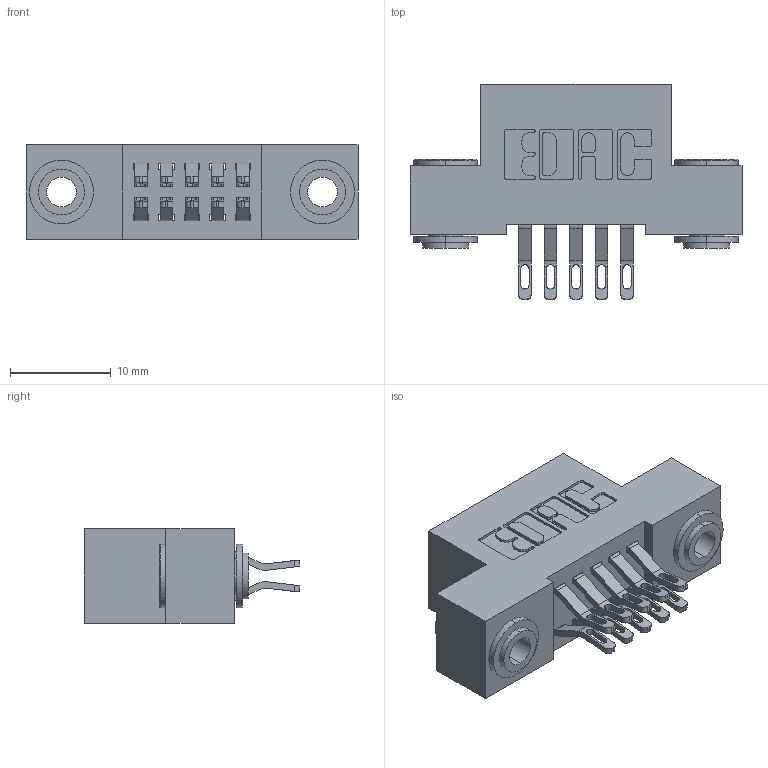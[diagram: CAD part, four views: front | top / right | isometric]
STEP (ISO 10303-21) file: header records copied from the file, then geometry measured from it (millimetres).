
FILE_DESCRIPTION (( 'STEP AP203' ), '1' );
FILE_NAME ('342-010-555-203.STEP', '2019-10-01T14:43:19', ( '' ), ( '' ), 'SwSTEP 2.0', 'SolidWorks 2016', '' );
FILE_SCHEMA (( 'CONFIG_CONTROL_DESIGN' ));
Length unit declared in the file: inch
Products named in the file (4): 342-010-555-203; 342 Part_.156 TH; 345-292-001_555 Tail; 342-250-002_345-250-002-102
Assembly tree (13 placements, depth 2):
  342-010-555-203
    342 Part_.156 TH
    345-292-001_555 Tail  x10
    342-250-002_345-250-002-102  x2
Bounding box: 33.02 x 21.47 x 9.4 mm (x, y, z)
Volume: 2842.3 mm3; surface area: 4025.7 mm2
Topology: 13 solids, 13 shells, 728 faces, 2205 edges, 1466 vertices
Faces by surface type: plane 416, cylinder 304, cone 8
Entity records: 8846 total; most frequent: CARTESIAN_POINT 1519, ORIENTED_EDGE 1418, DIRECTION 1367, EDGE_CURVE 709, LINE 537, VECTOR 537, VERTEX_POINT 470, AXIS2_PLACEMENT_3D 415
